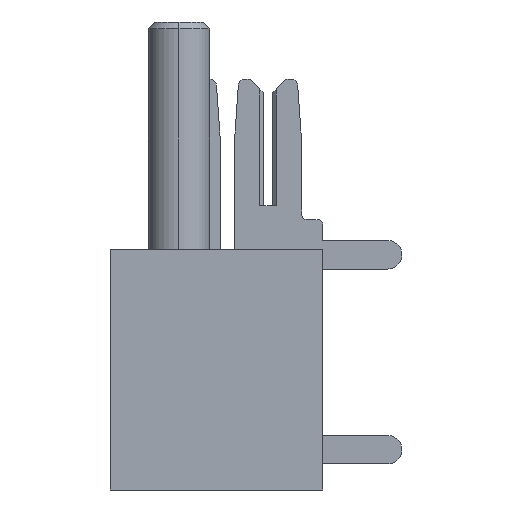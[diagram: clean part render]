
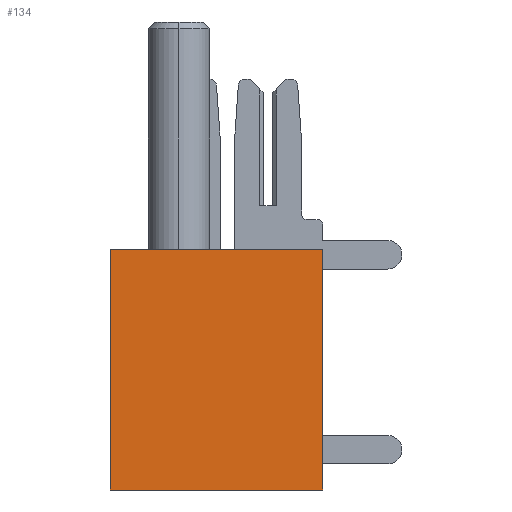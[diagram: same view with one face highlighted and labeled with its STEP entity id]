
A CAD part, left-side view. The second image highlights one B-rep face of the part: STEP entity #134.
In plain terms, the highlighted planar face has unit normal (-1, 0, 0).
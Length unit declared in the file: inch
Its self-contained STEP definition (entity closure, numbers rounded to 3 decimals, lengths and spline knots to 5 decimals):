
#134 = ADVANCED_FACE ( 'NONE', ( #4557 ), #6994, .T. ) ;
#1225 = EDGE_LOOP ( 'NONE', ( #5149, #10825, #4539, #6375 ) ) ;
#1381 = CARTESIAN_POINT ( 'NONE',  ( 0., 0.327, -0.37 ) ) ;
#1872 = DIRECTION ( 'NONE',  ( 0., 0., 1. ) ) ;
#2217 = VECTOR ( 'NONE', #6118, 39.37008 ) ;
#2854 = AXIS2_PLACEMENT_3D ( 'NONE', #4924, #5969, #1872 ) ;
#2911 = LINE ( 'NONE', #4745, #4688 ) ;
#3142 = LINE ( 'NONE', #12918, #6217 ) ;
#4539 = ORIENTED_EDGE ( 'NONE', *, *, #12758, .T. ) ;
#4550 = CARTESIAN_POINT ( 'NONE',  ( 0., 0., -0.37 ) ) ;
#4557 = FACE_OUTER_BOUND ( 'NONE', #1225, .T. ) ;
#4688 = VECTOR ( 'NONE', #9920, 39.37008 ) ;
#4745 = CARTESIAN_POINT ( 'NONE',  ( 0., 0., -0.37 ) ) ;
#4924 = CARTESIAN_POINT ( 'NONE',  ( 0., 0., -0.37 ) ) ;
#4940 = LINE ( 'NONE', #6160, #2217 ) ;
#4982 = VERTEX_POINT ( 'NONE', #4550 ) ;
#5079 = DIRECTION ( 'NONE',  ( 0., 0., 1. ) ) ;
#5119 = CARTESIAN_POINT ( 'NONE',  ( 0., 0.327, -0.37 ) ) ;
#5149 = ORIENTED_EDGE ( 'NONE', *, *, #11633, .F. ) ;
#5837 = EDGE_CURVE ( 'NONE', #4982, #5894, #3142, .T. ) ;
#5894 = VERTEX_POINT ( 'NONE', #8891 ) ;
#5969 = DIRECTION ( 'NONE',  ( -1., 0., 0. ) ) ;
#6118 = DIRECTION ( 'NONE',  ( 0., -1., 0. ) ) ;
#6160 = CARTESIAN_POINT ( 'NONE',  ( 0., 0., 0. ) ) ;
#6217 = VECTOR ( 'NONE', #6802, 39.37008 ) ;
#6375 = ORIENTED_EDGE ( 'NONE', *, *, #5837, .T. ) ;
#6802 = DIRECTION ( 'NONE',  ( 0., 0., 1. ) ) ;
#6994 = PLANE ( 'NONE',  #2854 ) ;
#7925 = EDGE_CURVE ( 'NONE', #10198, #10102, #11321, .T. ) ;
#7947 = VECTOR ( 'NONE', #5079, 39.37008 ) ;
#8593 = CARTESIAN_POINT ( 'NONE',  ( 0., 0.327, 0. ) ) ;
#8891 = CARTESIAN_POINT ( 'NONE',  ( 0., 0., 0. ) ) ;
#9920 = DIRECTION ( 'NONE',  ( 0., -1., 0. ) ) ;
#10102 = VERTEX_POINT ( 'NONE', #8593 ) ;
#10198 = VERTEX_POINT ( 'NONE', #1381 ) ;
#10825 = ORIENTED_EDGE ( 'NONE', *, *, #7925, .F. ) ;
#11321 = LINE ( 'NONE', #5119, #7947 ) ;
#11633 = EDGE_CURVE ( 'NONE', #10102, #5894, #4940, .T. ) ;
#12758 = EDGE_CURVE ( 'NONE', #10198, #4982, #2911, .T. ) ;
#12918 = CARTESIAN_POINT ( 'NONE',  ( 0., 0., -0.37 ) ) ;
